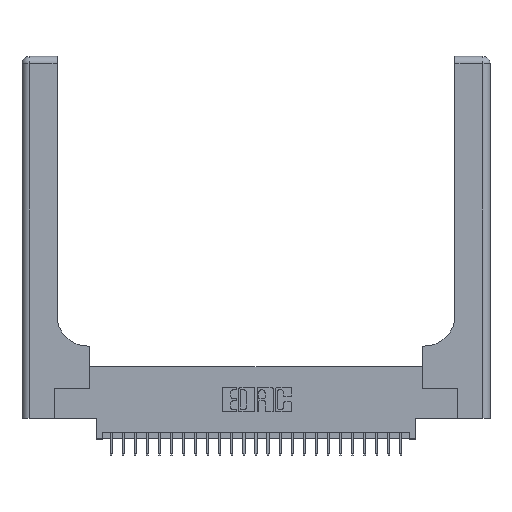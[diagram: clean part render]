
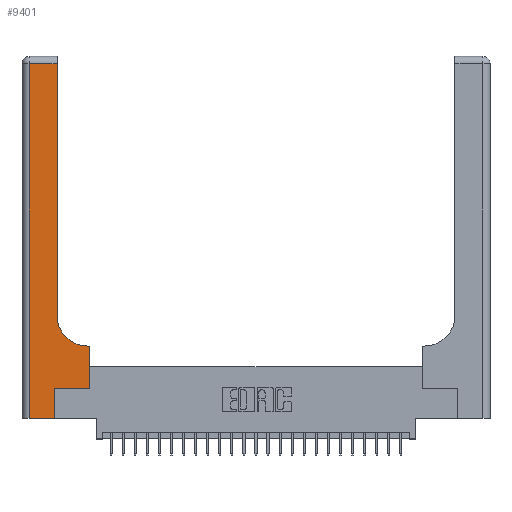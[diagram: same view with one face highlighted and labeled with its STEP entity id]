
A CAD part, top view. The second image highlights one B-rep face of the part: STEP entity #9401.
In plain terms, the highlighted planar face has unit normal (0, 0, 1).
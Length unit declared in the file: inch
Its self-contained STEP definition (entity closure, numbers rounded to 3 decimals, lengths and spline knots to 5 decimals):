
#47 = LINE ( 'NONE', #16124, #10035 ) ;
#190 = CARTESIAN_POINT ( 'NONE',  ( 0., 2.94, 0.37 ) ) ;
#1075 = VECTOR ( 'NONE', #26851, 39.37008 ) ;
#1192 = ORIENTED_EDGE ( 'NONE', *, *, #6338, .T. ) ;
#1292 = CARTESIAN_POINT ( 'NONE',  ( 0.06, 3., 0.37 ) ) ;
#2622 = CARTESIAN_POINT ( 'NONE',  ( 0.269, 0.25, 0.37 ) ) ;
#2785 = CARTESIAN_POINT ( 'NONE',  ( 0.2915, 2.94, 0.37 ) ) ;
#3050 = DIRECTION ( 'NONE',  ( 0., 1., 0. ) ) ;
#3238 = VECTOR ( 'NONE', #10374, 39.37008 ) ;
#4004 = ORIENTED_EDGE ( 'NONE', *, *, #15895, .T. ) ;
#4074 = AXIS2_PLACEMENT_3D ( 'NONE', #23532, #19141, #4328 ) ;
#4130 = ORIENTED_EDGE ( 'NONE', *, *, #10917, .T. ) ;
#4222 = CIRCLE ( 'NONE', #13518, 0.25 ) ;
#4328 = DIRECTION ( 'NONE',  ( -1., 0., 0. ) ) ;
#4383 = CARTESIAN_POINT ( 'NONE',  ( 0.2915, 0.6, 0.37 ) ) ;
#5232 = VERTEX_POINT ( 'NONE', #21137 ) ;
#5479 = EDGE_CURVE ( 'NONE', #7686, #5836, #6530, .T. ) ;
#5575 = CARTESIAN_POINT ( 'NONE',  ( 0.5415, 0.85, 0.37 ) ) ;
#5787 = CARTESIAN_POINT ( 'NONE',  ( 0.2915, 3., 0.37 ) ) ;
#5836 = VERTEX_POINT ( 'NONE', #8339 ) ;
#5920 = CARTESIAN_POINT ( 'NONE',  ( 0.06, 0., 0.37 ) ) ;
#6338 = EDGE_CURVE ( 'NONE', #9151, #11891, #27066, .T. ) ;
#6530 = LINE ( 'NONE', #2622, #8973 ) ;
#7098 = VECTOR ( 'NONE', #16637, 39.37008 ) ;
#7310 = EDGE_CURVE ( 'NONE', #20521, #27213, #10031, .T. ) ;
#7686 = VERTEX_POINT ( 'NONE', #23892 ) ;
#7709 = VERTEX_POINT ( 'NONE', #23761 ) ;
#8339 = CARTESIAN_POINT ( 'NONE',  ( 0.5585, 0.25, 0.37 ) ) ;
#8384 = ORIENTED_EDGE ( 'NONE', *, *, #7310, .T. ) ;
#8874 = EDGE_CURVE ( 'NONE', #7709, #9151, #4222, .T. ) ;
#8895 = LINE ( 'NONE', #190, #20412 ) ;
#8973 = VECTOR ( 'NONE', #23756, 39.37008 ) ;
#9056 = PLANE ( 'NONE',  #4074 ) ;
#9151 = VERTEX_POINT ( 'NONE', #23328 ) ;
#9212 = DIRECTION ( 'NONE',  ( 1., 0., 0. ) ) ;
#9401 = ADVANCED_FACE ( 'NONE', ( #21604 ), #9056, .F. ) ;
#9493 = DIRECTION ( 'NONE',  ( 0., 0., -1. ) ) ;
#10031 = LINE ( 'NONE', #1292, #1075 ) ;
#10035 = VECTOR ( 'NONE', #18454, 39.37008 ) ;
#10374 = DIRECTION ( 'NONE',  ( 0., 1., 0. ) ) ;
#10680 = ORIENTED_EDGE ( 'NONE', *, *, #21890, .T. ) ;
#10917 = EDGE_CURVE ( 'NONE', #27213, #5232, #18705, .T. ) ;
#11227 = ORIENTED_EDGE ( 'NONE', *, *, #8874, .T. ) ;
#11891 = VERTEX_POINT ( 'NONE', #2785 ) ;
#13518 = AXIS2_PLACEMENT_3D ( 'NONE', #5575, #9493, #9212 ) ;
#14568 = VECTOR ( 'NONE', #25491, 39.37008 ) ;
#15895 = EDGE_CURVE ( 'NONE', #16227, #7709, #27202, .T. ) ;
#16048 = LINE ( 'NONE', #26242, #22328 ) ;
#16124 = CARTESIAN_POINT ( 'NONE',  ( 0.269, 0., 0.37 ) ) ;
#16227 = VERTEX_POINT ( 'NONE', #21722 ) ;
#16275 = EDGE_CURVE ( 'NONE', #11891, #20521, #8895, .T. ) ;
#16637 = DIRECTION ( 'NONE',  ( 1., 0., 0. ) ) ;
#17311 = DIRECTION ( 'NONE',  ( -1., 0., 0. ) ) ;
#18454 = DIRECTION ( 'NONE',  ( 0., 1., 0. ) ) ;
#18705 = LINE ( 'NONE', #27132, #7098 ) ;
#19141 = DIRECTION ( 'NONE',  ( 0., 0., -1. ) ) ;
#20412 = VECTOR ( 'NONE', #17311, 39.37008 ) ;
#20521 = VERTEX_POINT ( 'NONE', #23568 ) ;
#21137 = CARTESIAN_POINT ( 'NONE',  ( 0.269, 0., 0.37 ) ) ;
#21477 = EDGE_LOOP ( 'NONE', ( #1192, #23607, #8384, #4130, #27241, #26535, #10680, #4004, #11227 ) ) ;
#21604 = FACE_OUTER_BOUND ( 'NONE', #21477, .T. ) ;
#21722 = CARTESIAN_POINT ( 'NONE',  ( 0.5585, 0.6, 0.37 ) ) ;
#21890 = EDGE_CURVE ( 'NONE', #5836, #16227, #16048, .T. ) ;
#22328 = VECTOR ( 'NONE', #3050, 39.37008 ) ;
#23023 = EDGE_CURVE ( 'NONE', #5232, #7686, #47, .T. ) ;
#23328 = CARTESIAN_POINT ( 'NONE',  ( 0.2915, 0.85, 0.37 ) ) ;
#23532 = CARTESIAN_POINT ( 'NONE',  ( 0., 3., 0.37 ) ) ;
#23568 = CARTESIAN_POINT ( 'NONE',  ( 0.06, 2.94, 0.37 ) ) ;
#23607 = ORIENTED_EDGE ( 'NONE', *, *, #16275, .T. ) ;
#23756 = DIRECTION ( 'NONE',  ( 1., 0., 0. ) ) ;
#23761 = CARTESIAN_POINT ( 'NONE',  ( 0.5415, 0.6, 0.37 ) ) ;
#23892 = CARTESIAN_POINT ( 'NONE',  ( 0.269, 0.25, 0.37 ) ) ;
#25491 = DIRECTION ( 'NONE',  ( -1., 0., 0. ) ) ;
#26242 = CARTESIAN_POINT ( 'NONE',  ( 0.5585, 0.25, 0.37 ) ) ;
#26535 = ORIENTED_EDGE ( 'NONE', *, *, #5479, .T. ) ;
#26851 = DIRECTION ( 'NONE',  ( 0., -1., 0. ) ) ;
#27066 = LINE ( 'NONE', #5787, #3238 ) ;
#27132 = CARTESIAN_POINT ( 'NONE',  ( 0., 0., 0.37 ) ) ;
#27202 = LINE ( 'NONE', #4383, #14568 ) ;
#27213 = VERTEX_POINT ( 'NONE', #5920 ) ;
#27241 = ORIENTED_EDGE ( 'NONE', *, *, #23023, .T. ) ;
